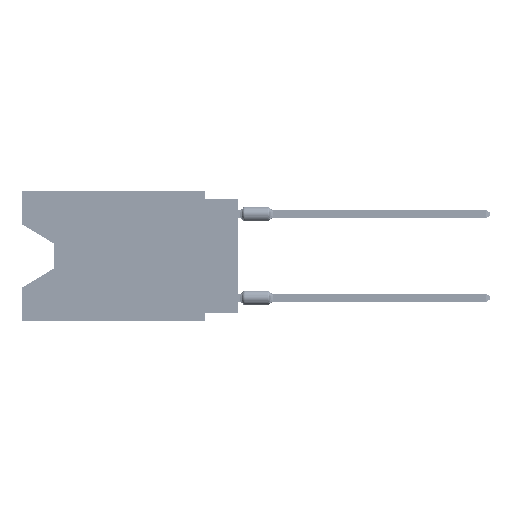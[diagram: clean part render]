
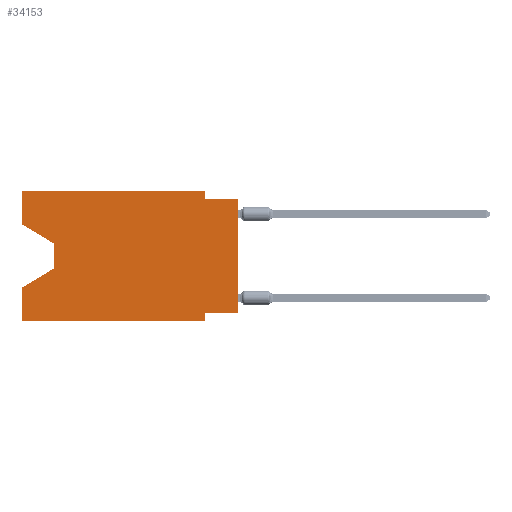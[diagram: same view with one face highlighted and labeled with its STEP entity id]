
A CAD part, left-side view. The second image highlights one B-rep face of the part: STEP entity #34153.
In plain terms, the highlighted planar face has unit normal (-1, 0, 0).
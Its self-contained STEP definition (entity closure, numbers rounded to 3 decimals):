
#2124 = ORIENTED_EDGE ( 'NONE', *, *, #63772, .F. ) ;
#2281 = LINE ( 'NONE', #24445, #71086 ) ;
#2543 = CARTESIAN_POINT ( 'NONE',  ( 0., 16.383, -2.546 ) ) ;
#2677 = VERTEX_POINT ( 'NONE', #19335 ) ;
#3522 = CARTESIAN_POINT ( 'NONE',  ( 0., 16.383, -9.906 ) ) ;
#4327 = LINE ( 'NONE', #70478, #20070 ) ;
#5218 = VERTEX_POINT ( 'NONE', #68023 ) ;
#6708 = LINE ( 'NONE', #61606, #24070 ) ;
#7888 = ORIENTED_EDGE ( 'NONE', *, *, #23505, .T. ) ;
#8416 = CARTESIAN_POINT ( 'NONE',  ( 0., 0., 0. ) ) ;
#9685 = VERTEX_POINT ( 'NONE', #17580 ) ;
#9836 = EDGE_LOOP ( 'NONE', ( #31973, #24657, #52308, #43378, #7888, #65652, #31874, #56835, #10825, #58098, #56817, #2124 ) ) ;
#10312 = LINE ( 'NONE', #45798, #68697 ) ;
#10825 = ORIENTED_EDGE ( 'NONE', *, *, #60176, .F. ) ;
#12063 = VERTEX_POINT ( 'NONE', #15887 ) ;
#12185 = CARTESIAN_POINT ( 'NONE',  ( 0., 2.54, -9.906 ) ) ;
#13382 = CARTESIAN_POINT ( 'NONE',  ( 0., 16.383, 0. ) ) ;
#13726 = EDGE_CURVE ( 'NONE', #48854, #12063, #2281, .T. ) ;
#14348 = EDGE_CURVE ( 'NONE', #9685, #44307, #4327, .T. ) ;
#15887 = CARTESIAN_POINT ( 'NONE',  ( 0., 16.383, -7.36 ) ) ;
#16123 = CARTESIAN_POINT ( 'NONE',  ( 0., 2.54, -9.271 ) ) ;
#16470 = DIRECTION ( 'NONE',  ( 0., -0.855, -0.519 ) ) ;
#17478 = CARTESIAN_POINT ( 'NONE',  ( 0., 2.54, 0. ) ) ;
#17580 = CARTESIAN_POINT ( 'NONE',  ( 0., 16.383, 0. ) ) ;
#17638 = LINE ( 'NONE', #12185, #27862 ) ;
#17866 = VERTEX_POINT ( 'NONE', #16123 ) ;
#19335 = CARTESIAN_POINT ( 'NONE',  ( 0., 2.54, -9.906 ) ) ;
#20070 = VECTOR ( 'NONE', #52701, 1000. ) ;
#20327 = EDGE_CURVE ( 'NONE', #48228, #12063, #68984, .T. ) ;
#21283 = CARTESIAN_POINT ( 'NONE',  ( 0., 16.383, 0. ) ) ;
#23119 = VERTEX_POINT ( 'NONE', #2543 ) ;
#23505 = EDGE_CURVE ( 'NONE', #48228, #2677, #58419, .T. ) ;
#24070 = VECTOR ( 'NONE', #56860, 1000. ) ;
#24445 = CARTESIAN_POINT ( 'NONE',  ( 0., 13.97, -5.893 ) ) ;
#24586 = VERTEX_POINT ( 'NONE', #31701 ) ;
#24657 = ORIENTED_EDGE ( 'NONE', *, *, #43472, .T. ) ;
#25421 = LINE ( 'NONE', #66365, #54408 ) ;
#25774 = DIRECTION ( 'NONE',  ( 0., 0., -1. ) ) ;
#26072 = DIRECTION ( 'NONE',  ( 0., 1., 0. ) ) ;
#27862 = VECTOR ( 'NONE', #44905, 1000. ) ;
#27969 = EDGE_CURVE ( 'NONE', #17866, #2677, #17638, .T. ) ;
#28445 = DIRECTION ( 'NONE',  ( 1., 0., 0. ) ) ;
#29187 = CARTESIAN_POINT ( 'NONE',  ( 0., 2.54, 0. ) ) ;
#30104 = VECTOR ( 'NONE', #66364, 1000. ) ;
#30445 = DIRECTION ( 'NONE',  ( 0., -1., 0. ) ) ;
#31701 = CARTESIAN_POINT ( 'NONE',  ( 0., 0., -0.635 ) ) ;
#31851 = LINE ( 'NONE', #21283, #30104 ) ;
#31874 = ORIENTED_EDGE ( 'NONE', *, *, #59628, .F. ) ;
#31973 = ORIENTED_EDGE ( 'NONE', *, *, #70927, .T. ) ;
#32122 = EDGE_CURVE ( 'NONE', #44307, #54149, #68437, .T. ) ;
#34153 = ADVANCED_FACE ( 'NONE', ( #50617 ), #61539, .F. ) ;
#34611 = CARTESIAN_POINT ( 'NONE',  ( 0., 16.383, 0. ) ) ;
#35301 = DIRECTION ( 'NONE',  ( 0., 0., 1. ) ) ;
#40803 = DIRECTION ( 'NONE',  ( 0., 0., -1. ) ) ;
#41512 = DIRECTION ( 'NONE',  ( 0., 0.855, -0.519 ) ) ;
#42166 = VERTEX_POINT ( 'NONE', #69300 ) ;
#43060 = CARTESIAN_POINT ( 'NONE',  ( 0., 16.383, -9.906 ) ) ;
#43378 = ORIENTED_EDGE ( 'NONE', *, *, #20327, .F. ) ;
#43472 = EDGE_CURVE ( 'NONE', #42166, #48854, #25421, .T. ) ;
#43585 = CARTESIAN_POINT ( 'NONE',  ( 0., 2.54, -0.635 ) ) ;
#44307 = VERTEX_POINT ( 'NONE', #17478 ) ;
#44669 = AXIS2_PLACEMENT_3D ( 'NONE', #34611, #28445, #55726 ) ;
#44905 = DIRECTION ( 'NONE',  ( 0., 0., -1. ) ) ;
#45798 = CARTESIAN_POINT ( 'NONE',  ( 0., 16.383, -2.546 ) ) ;
#48228 = VERTEX_POINT ( 'NONE', #43060 ) ;
#48854 = VERTEX_POINT ( 'NONE', #56274 ) ;
#48965 = LINE ( 'NONE', #54790, #51896 ) ;
#50617 = FACE_OUTER_BOUND ( 'NONE', #9836, .T. ) ;
#51896 = VECTOR ( 'NONE', #26072, 1000. ) ;
#52308 = ORIENTED_EDGE ( 'NONE', *, *, #13726, .T. ) ;
#52701 = DIRECTION ( 'NONE',  ( 0., -1., 0. ) ) ;
#54149 = VERTEX_POINT ( 'NONE', #43585 ) ;
#54408 = VECTOR ( 'NONE', #25774, 1000. ) ;
#54790 = CARTESIAN_POINT ( 'NONE',  ( 0., 0., -9.271 ) ) ;
#55726 = DIRECTION ( 'NONE',  ( 0., 0., -1. ) ) ;
#56274 = CARTESIAN_POINT ( 'NONE',  ( 0., 13.97, -5.893 ) ) ;
#56817 = ORIENTED_EDGE ( 'NONE', *, *, #14348, .F. ) ;
#56835 = ORIENTED_EDGE ( 'NONE', *, *, #64796, .T. ) ;
#56860 = DIRECTION ( 'NONE',  ( 0., -1., 0. ) ) ;
#58058 = VECTOR ( 'NONE', #35301, 1000. ) ;
#58098 = ORIENTED_EDGE ( 'NONE', *, *, #32122, .F. ) ;
#58419 = LINE ( 'NONE', #3522, #70547 ) ;
#59628 = EDGE_CURVE ( 'NONE', #5218, #17866, #48965, .T. ) ;
#60176 = EDGE_CURVE ( 'NONE', #54149, #24586, #6708, .T. ) ;
#60745 = VECTOR ( 'NONE', #40803, 1000. ) ;
#61539 = PLANE ( 'NONE',  #44669 ) ;
#61606 = CARTESIAN_POINT ( 'NONE',  ( 0., 0., -0.635 ) ) ;
#63283 = LINE ( 'NONE', #8416, #58058 ) ;
#63772 = EDGE_CURVE ( 'NONE', #23119, #9685, #31851, .T. ) ;
#64796 = EDGE_CURVE ( 'NONE', #5218, #24586, #63283, .T. ) ;
#65652 = ORIENTED_EDGE ( 'NONE', *, *, #27969, .F. ) ;
#65915 = VECTOR ( 'NONE', #68275, 1000. ) ;
#66364 = DIRECTION ( 'NONE',  ( 0., 0., 1. ) ) ;
#66365 = CARTESIAN_POINT ( 'NONE',  ( 0., 13.97, -4.013 ) ) ;
#68023 = CARTESIAN_POINT ( 'NONE',  ( 0., 0., -9.271 ) ) ;
#68275 = DIRECTION ( 'NONE',  ( 0., 0., 1. ) ) ;
#68437 = LINE ( 'NONE', #29187, #60745 ) ;
#68697 = VECTOR ( 'NONE', #16470, 1000. ) ;
#68984 = LINE ( 'NONE', #13382, #65915 ) ;
#69300 = CARTESIAN_POINT ( 'NONE',  ( 0., 13.97, -4.013 ) ) ;
#70478 = CARTESIAN_POINT ( 'NONE',  ( 0., 16.383, 0. ) ) ;
#70547 = VECTOR ( 'NONE', #30445, 1000. ) ;
#70927 = EDGE_CURVE ( 'NONE', #23119, #42166, #10312, .T. ) ;
#71086 = VECTOR ( 'NONE', #41512, 1000. ) ;
